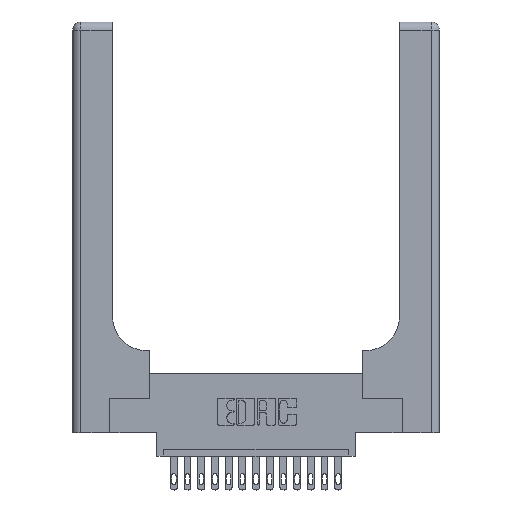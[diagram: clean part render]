
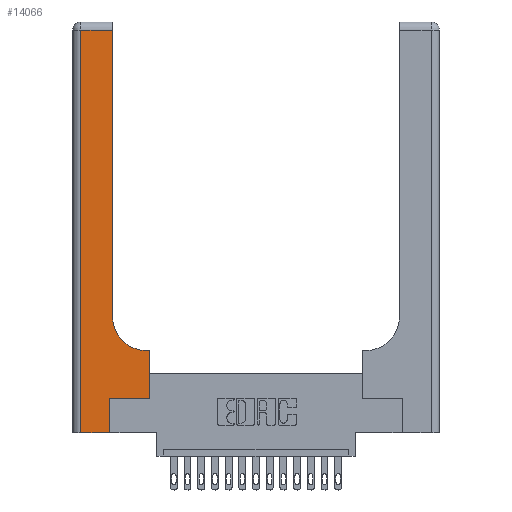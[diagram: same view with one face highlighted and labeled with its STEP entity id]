
A CAD part, top view. The second image highlights one B-rep face of the part: STEP entity #14066.
In plain terms, the highlighted planar face has unit normal (0, 0, 1).
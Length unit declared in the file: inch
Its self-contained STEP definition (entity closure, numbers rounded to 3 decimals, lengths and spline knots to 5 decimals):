
#27 = LINE ( 'NONE', #9733, #12581 ) ;
#495 = LINE ( 'NONE', #8394, #11681 ) ;
#559 = CARTESIAN_POINT ( 'NONE',  ( 0.269, 0.25, 0.37 ) ) ;
#660 = EDGE_LOOP ( 'NONE', ( #14168, #18046, #8427, #2954, #7655, #13095, #13418, #7902, #11325 ) ) ;
#700 = EDGE_CURVE ( 'NONE', #7465, #11642, #10393, .T. ) ;
#833 = VERTEX_POINT ( 'NONE', #17724 ) ;
#1133 = LINE ( 'NONE', #15290, #12084 ) ;
#1295 = DIRECTION ( 'NONE',  ( 0., 1., 0. ) ) ;
#1818 = EDGE_CURVE ( 'NONE', #16467, #3827, #15100, .T. ) ;
#1885 = CARTESIAN_POINT ( 'NONE',  ( 0.5585, 0.25, 0.37 ) ) ;
#1966 = CARTESIAN_POINT ( 'NONE',  ( 0.2915, 2.94, 0.37 ) ) ;
#1998 = VERTEX_POINT ( 'NONE', #9332 ) ;
#2381 = DIRECTION ( 'NONE',  ( 1., 0., 0. ) ) ;
#2954 = ORIENTED_EDGE ( 'NONE', *, *, #5789, .T. ) ;
#3646 = AXIS2_PLACEMENT_3D ( 'NONE', #7614, #6154, #17820 ) ;
#3824 = CARTESIAN_POINT ( 'NONE',  ( 0.2915, 0.6, 0.37 ) ) ;
#3827 = VERTEX_POINT ( 'NONE', #14405 ) ;
#4163 = AXIS2_PLACEMENT_3D ( 'NONE', #11927, #7586, #17915 ) ;
#4299 = LINE ( 'NONE', #3824, #6582 ) ;
#4340 = EDGE_CURVE ( 'NONE', #3827, #5059, #13559, .T. ) ;
#5059 = VERTEX_POINT ( 'NONE', #1966 ) ;
#5683 = LINE ( 'NONE', #6073, #16866 ) ;
#5789 = EDGE_CURVE ( 'NONE', #10387, #1998, #495, .T. ) ;
#5817 = EDGE_CURVE ( 'NONE', #833, #10387, #27, .T. ) ;
#6073 = CARTESIAN_POINT ( 'NONE',  ( 0.5585, 0.25, 0.37 ) ) ;
#6154 = DIRECTION ( 'NONE',  ( 0., 0., -1. ) ) ;
#6582 = VECTOR ( 'NONE', #18431, 39.37008 ) ;
#6988 = EDGE_CURVE ( 'NONE', #5059, #833, #1133, .T. ) ;
#7295 = CARTESIAN_POINT ( 'NONE',  ( 0.2915, 3., 0.37 ) ) ;
#7465 = VERTEX_POINT ( 'NONE', #14501 ) ;
#7586 = DIRECTION ( 'NONE',  ( 0., 0., -1. ) ) ;
#7614 = CARTESIAN_POINT ( 'NONE',  ( 0.5415, 0.85, 0.37 ) ) ;
#7632 = CARTESIAN_POINT ( 'NONE',  ( 0.269, 0., 0.37 ) ) ;
#7655 = ORIENTED_EDGE ( 'NONE', *, *, #10780, .T. ) ;
#7704 = VERTEX_POINT ( 'NONE', #10845 ) ;
#7902 = ORIENTED_EDGE ( 'NONE', *, *, #15154, .T. ) ;
#8394 = CARTESIAN_POINT ( 'NONE',  ( 0., 0., 0.37 ) ) ;
#8427 = ORIENTED_EDGE ( 'NONE', *, *, #5817, .T. ) ;
#8951 = CARTESIAN_POINT ( 'NONE',  ( 0.5415, 0.6, 0.37 ) ) ;
#9332 = CARTESIAN_POINT ( 'NONE',  ( 0.269, 0., 0.37 ) ) ;
#9733 = CARTESIAN_POINT ( 'NONE',  ( 0.06, 3., 0.37 ) ) ;
#9800 = DIRECTION ( 'NONE',  ( 0., -1., 0. ) ) ;
#9948 = LINE ( 'NONE', #7632, #18150 ) ;
#10387 = VERTEX_POINT ( 'NONE', #17041 ) ;
#10393 = LINE ( 'NONE', #559, #16091 ) ;
#10577 = DIRECTION ( 'NONE',  ( 0., 1., 0. ) ) ;
#10780 = EDGE_CURVE ( 'NONE', #1998, #7465, #9948, .T. ) ;
#10845 = CARTESIAN_POINT ( 'NONE',  ( 0.5585, 0.6, 0.37 ) ) ;
#11325 = ORIENTED_EDGE ( 'NONE', *, *, #1818, .T. ) ;
#11642 = VERTEX_POINT ( 'NONE', #1885 ) ;
#11681 = VECTOR ( 'NONE', #2381, 39.37008 ) ;
#11927 = CARTESIAN_POINT ( 'NONE',  ( 0., 3., 0.37 ) ) ;
#12084 = VECTOR ( 'NONE', #12603, 39.37008 ) ;
#12581 = VECTOR ( 'NONE', #9800, 39.37008 ) ;
#12603 = DIRECTION ( 'NONE',  ( -1., 0., 0. ) ) ;
#12763 = FACE_OUTER_BOUND ( 'NONE', #660, .T. ) ;
#13095 = ORIENTED_EDGE ( 'NONE', *, *, #700, .T. ) ;
#13380 = DIRECTION ( 'NONE',  ( 0., 1., 0. ) ) ;
#13418 = ORIENTED_EDGE ( 'NONE', *, *, #14881, .T. ) ;
#13559 = LINE ( 'NONE', #7295, #15602 ) ;
#13891 = DIRECTION ( 'NONE',  ( 1., 0., 0. ) ) ;
#14066 = ADVANCED_FACE ( 'NONE', ( #12763 ), #16394, .F. ) ;
#14168 = ORIENTED_EDGE ( 'NONE', *, *, #4340, .T. ) ;
#14405 = CARTESIAN_POINT ( 'NONE',  ( 0.2915, 0.85, 0.37 ) ) ;
#14501 = CARTESIAN_POINT ( 'NONE',  ( 0.269, 0.25, 0.37 ) ) ;
#14881 = EDGE_CURVE ( 'NONE', #11642, #7704, #5683, .T. ) ;
#15100 = CIRCLE ( 'NONE', #3646, 0.25 ) ;
#15154 = EDGE_CURVE ( 'NONE', #7704, #16467, #4299, .T. ) ;
#15290 = CARTESIAN_POINT ( 'NONE',  ( 0., 2.94, 0.37 ) ) ;
#15602 = VECTOR ( 'NONE', #1295, 39.37008 ) ;
#16091 = VECTOR ( 'NONE', #13891, 39.37008 ) ;
#16394 = PLANE ( 'NONE',  #4163 ) ;
#16467 = VERTEX_POINT ( 'NONE', #8951 ) ;
#16866 = VECTOR ( 'NONE', #13380, 39.37008 ) ;
#17041 = CARTESIAN_POINT ( 'NONE',  ( 0.06, 0., 0.37 ) ) ;
#17724 = CARTESIAN_POINT ( 'NONE',  ( 0.06, 2.94, 0.37 ) ) ;
#17820 = DIRECTION ( 'NONE',  ( 1., 0., 0. ) ) ;
#17915 = DIRECTION ( 'NONE',  ( -1., 0., 0. ) ) ;
#18046 = ORIENTED_EDGE ( 'NONE', *, *, #6988, .T. ) ;
#18150 = VECTOR ( 'NONE', #10577, 39.37008 ) ;
#18431 = DIRECTION ( 'NONE',  ( -1., 0., 0. ) ) ;
